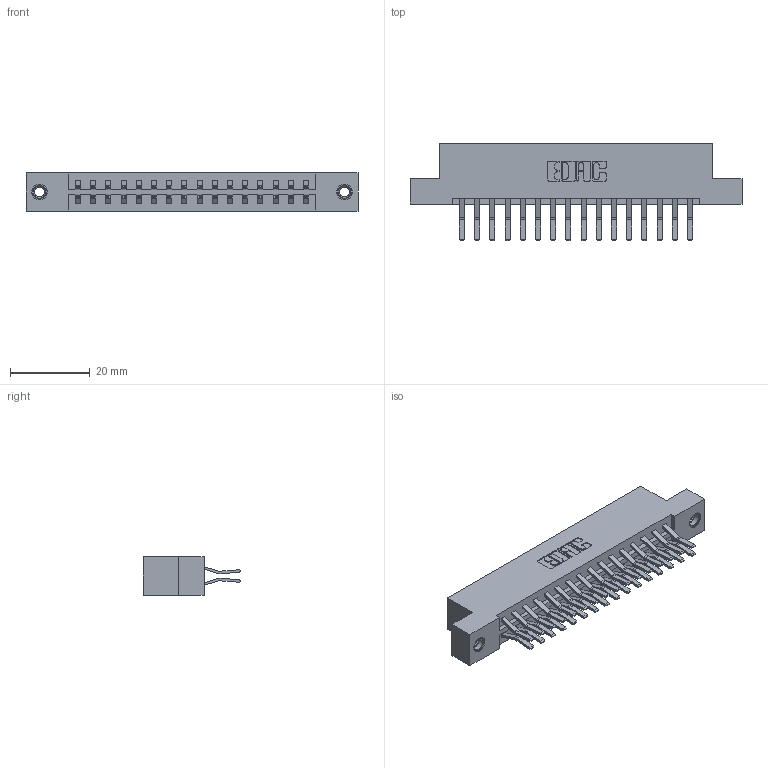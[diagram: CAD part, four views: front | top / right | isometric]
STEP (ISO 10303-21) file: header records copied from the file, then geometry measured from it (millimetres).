
FILE_DESCRIPTION (( 'STEP AP203' ), '1' );
FILE_NAME ('379-032-560-207.STEP', '2020-09-30T17:33:26', ( '' ), ( '' ), 'SwSTEP 2.0', 'SolidWorks 2020', '' );
FILE_SCHEMA (( 'CONFIG_CONTROL_DESIGN' ));
Length unit declared in the file: inch
Products named in the file (4): 345-292-001_560 Tail; 345-250-001_345-250-005-103; 379 Part_Flush - .156 Dia - TI; 379-032-560-207
Assembly tree (35 placements, depth 2):
  379-032-560-207
    379 Part_Flush - .156 Dia - TI
    345-292-001_560 Tail  x32
    345-250-001_345-250-005-103  x2
Bounding box: 83.19 x 24.45 x 9.53 mm (x, y, z)
Volume: 8731.2 mm3; surface area: 10212 mm2
Topology: 35 solids, 35 shells, 1902 faces, 5599 edges, 3682 vertices
Faces by surface type: plane 1254, cylinder 632, cone 12, torus 4
Entity records: 14930 total; most frequent: CARTESIAN_POINT 2489, ORIENTED_EDGE 2418, DIRECTION 2207, EDGE_CURVE 1209, LINE 1057, VECTOR 1057, VERTEX_POINT 800, AXIS2_PLACEMENT_3D 575
